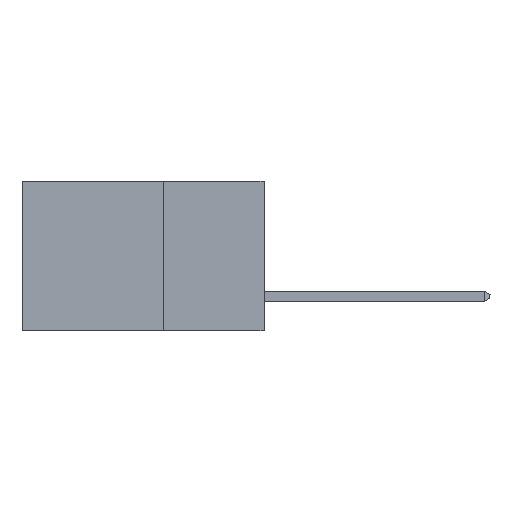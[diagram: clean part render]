
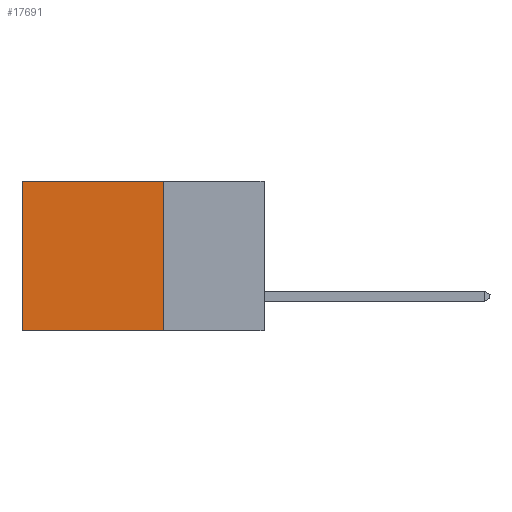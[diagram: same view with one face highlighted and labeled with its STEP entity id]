
A CAD part, left-side view. The second image highlights one B-rep face of the part: STEP entity #17691.
In plain terms, the highlighted planar face has unit normal (-1, 0, 0).
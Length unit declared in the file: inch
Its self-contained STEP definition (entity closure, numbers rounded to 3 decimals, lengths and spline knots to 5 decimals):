
#686 = VECTOR ( 'NONE', #17734, 39.37008 ) ;
#927 = CARTESIAN_POINT ( 'NONE',  ( 0.2615, 0.25, 0. ) ) ;
#1458 = EDGE_LOOP ( 'NONE', ( #16623, #9703, #17989, #3749 ) ) ;
#1595 = VERTEX_POINT ( 'NONE', #14417 ) ;
#1919 = LINE ( 'NONE', #18421, #9125 ) ;
#2395 = CARTESIAN_POINT ( 'NONE',  ( 0.2615, 0.25, -0.37 ) ) ;
#2539 = VERTEX_POINT ( 'NONE', #12427 ) ;
#2702 = DIRECTION ( 'NONE',  ( 0., 1., 0. ) ) ;
#3306 = VECTOR ( 'NONE', #14154, 39.37008 ) ;
#3749 = ORIENTED_EDGE ( 'NONE', *, *, #4130, .T. ) ;
#3979 = EDGE_CURVE ( 'NONE', #1595, #10519, #1919, .T. ) ;
#4029 = LINE ( 'NONE', #2395, #3306 ) ;
#4130 = EDGE_CURVE ( 'NONE', #4528, #2539, #12808, .T. ) ;
#4524 = CARTESIAN_POINT ( 'NONE',  ( 0.2615, 0.6, -0.37 ) ) ;
#4528 = VERTEX_POINT ( 'NONE', #927 ) ;
#5127 = PLANE ( 'NONE',  #15727 ) ;
#5503 = CARTESIAN_POINT ( 'NONE',  ( 0.2615, 0.25, 0. ) ) ;
#6594 = CARTESIAN_POINT ( 'NONE',  ( 0.2615, 0.6, -0.37 ) ) ;
#9125 = VECTOR ( 'NONE', #17064, 39.37008 ) ;
#9566 = EDGE_CURVE ( 'NONE', #2539, #10519, #11828, .T. ) ;
#9703 = ORIENTED_EDGE ( 'NONE', *, *, #3979, .F. ) ;
#10519 = VERTEX_POINT ( 'NONE', #6594 ) ;
#11150 = FACE_OUTER_BOUND ( 'NONE', #1458, .T. ) ;
#11828 = LINE ( 'NONE', #4524, #686 ) ;
#12351 = CARTESIAN_POINT ( 'NONE',  ( 0.2615, 0.25, -0.37 ) ) ;
#12427 = CARTESIAN_POINT ( 'NONE',  ( 0.2615, 0.6, 0. ) ) ;
#12808 = LINE ( 'NONE', #5503, #14731 ) ;
#14154 = DIRECTION ( 'NONE',  ( 0., 0., -1. ) ) ;
#14417 = CARTESIAN_POINT ( 'NONE',  ( 0.2615, 0.25, -0.37 ) ) ;
#14731 = VECTOR ( 'NONE', #2702, 39.37008 ) ;
#15727 = AXIS2_PLACEMENT_3D ( 'NONE', #12351, #17076, #18251 ) ;
#16348 = EDGE_CURVE ( 'NONE', #4528, #1595, #4029, .T. ) ;
#16623 = ORIENTED_EDGE ( 'NONE', *, *, #9566, .T. ) ;
#17064 = DIRECTION ( 'NONE',  ( 0., 1., 0. ) ) ;
#17076 = DIRECTION ( 'NONE',  ( 1., 0., 0. ) ) ;
#17691 = ADVANCED_FACE ( 'NONE', ( #11150 ), #5127, .F. ) ;
#17734 = DIRECTION ( 'NONE',  ( 0., 0., -1. ) ) ;
#17989 = ORIENTED_EDGE ( 'NONE', *, *, #16348, .F. ) ;
#18251 = DIRECTION ( 'NONE',  ( 0., 0., -1. ) ) ;
#18421 = CARTESIAN_POINT ( 'NONE',  ( 0.2615, 0.25, -0.37 ) ) ;
